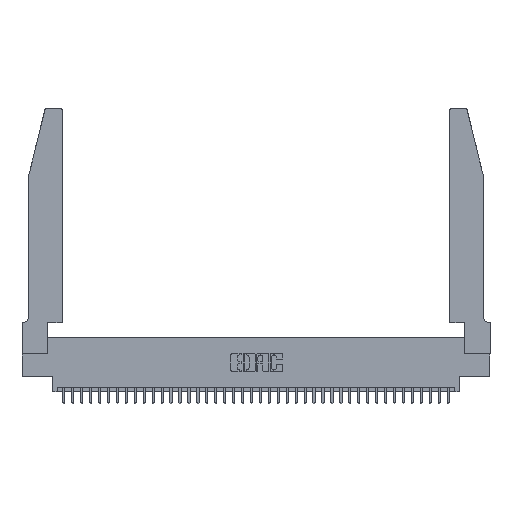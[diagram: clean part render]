
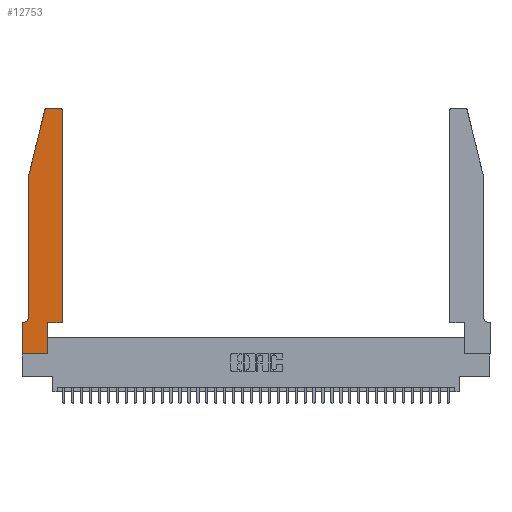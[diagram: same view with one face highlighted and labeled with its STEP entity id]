
A CAD part, top view. The second image highlights one B-rep face of the part: STEP entity #12753.
In plain terms, the highlighted planar face has unit normal (0, 0, 1).
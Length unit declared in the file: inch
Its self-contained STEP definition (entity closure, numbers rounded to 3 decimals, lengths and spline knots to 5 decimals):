
#182 = VECTOR ( 'NONE', #33319, 39.37008 ) ;
#279 = EDGE_CURVE ( 'NONE', #15512, #21603, #10615, .T. ) ;
#410 = DIRECTION ( 'NONE',  ( 1., 0., 0. ) ) ;
#689 = DIRECTION ( 'NONE',  ( 0., 0., 1. ) ) ;
#1297 = EDGE_CURVE ( 'NONE', #25329, #8774, #26705, .T. ) ;
#1304 = CARTESIAN_POINT ( 'NONE',  ( 0.0755, 2., 0.37 ) ) ;
#1874 = EDGE_CURVE ( 'NONE', #21657, #29614, #26146, .T. ) ;
#3122 = ORIENTED_EDGE ( 'NONE', *, *, #33252, .T. ) ;
#4706 = DIRECTION ( 'NONE',  ( 1., 0., 0. ) ) ;
#5196 = EDGE_LOOP ( 'NONE', ( #27425, #20992, #29736, #27773, #10238, #21027, #29947, #9993, #3122, #22848, #13541, #28700 ) ) ;
#5356 = DIRECTION ( 'NONE',  ( 1., 0., 0. ) ) ;
#5960 = AXIS2_PLACEMENT_3D ( 'NONE', #9141, #24368, #410 ) ;
#5963 = CARTESIAN_POINT ( 'NONE',  ( 0.0755, 0.35, 0.37 ) ) ;
#6253 = DIRECTION ( 'NONE',  ( 1., 0., 0. ) ) ;
#6362 = PLANE ( 'NONE',  #5960 ) ;
#7194 = CARTESIAN_POINT ( 'NONE',  ( 0.0755, 2., 0.37 ) ) ;
#7942 = VECTOR ( 'NONE', #10028, 39.37008 ) ;
#8774 = VERTEX_POINT ( 'NONE', #23199 ) ;
#9093 = CARTESIAN_POINT ( 'NONE',  ( 0., 0., 0.37 ) ) ;
#9141 = CARTESIAN_POINT ( 'NONE',  ( 0., 0.35, 0.37 ) ) ;
#9427 = CARTESIAN_POINT ( 'NONE',  ( 0.0755, 2., 0.37 ) ) ;
#9993 = ORIENTED_EDGE ( 'NONE', *, *, #1297, .T. ) ;
#10028 = DIRECTION ( 'NONE',  ( 0., 1., 0. ) ) ;
#10153 = CARTESIAN_POINT ( 'NONE',  ( 0.0755, 0.42, 0.37 ) ) ;
#10203 = AXIS2_PLACEMENT_3D ( 'NONE', #34656, #17429, #23490 ) ;
#10238 = ORIENTED_EDGE ( 'NONE', *, *, #11694, .T. ) ;
#10490 = VERTEX_POINT ( 'NONE', #22959 ) ;
#10532 = CARTESIAN_POINT ( 'NONE',  ( 0.2605, 2.75, 0.37 ) ) ;
#10615 = LINE ( 'NONE', #5963, #16751 ) ;
#11694 = EDGE_CURVE ( 'NONE', #26914, #15512, #14439, .T. ) ;
#11916 = DIRECTION ( 'NONE',  ( -1., 0., 0. ) ) ;
#12753 = ADVANCED_FACE ( 'NONE', ( #20498 ), #6362, .T. ) ;
#13520 = CARTESIAN_POINT ( 'NONE',  ( 0.0055, 0.35, 0.37 ) ) ;
#13541 = ORIENTED_EDGE ( 'NONE', *, *, #35552, .T. ) ;
#14439 = CIRCLE ( 'NONE', #10203, 0.07 ) ;
#15064 = DIRECTION ( 'NONE',  ( 1., 0., 0. ) ) ;
#15512 = VERTEX_POINT ( 'NONE', #13520 ) ;
#15790 = CARTESIAN_POINT ( 'NONE',  ( 0., 0., 0.37 ) ) ;
#15930 = VECTOR ( 'NONE', #25744, 39.37008 ) ;
#16115 = CARTESIAN_POINT ( 'NONE',  ( 0.4505, 0.35, 0.37 ) ) ;
#16228 = LINE ( 'NONE', #9427, #182 ) ;
#16472 = LINE ( 'NONE', #15790, #30693 ) ;
#16525 = VERTEX_POINT ( 'NONE', #7194 ) ;
#16751 = VECTOR ( 'NONE', #11916, 39.37008 ) ;
#16918 = LINE ( 'NONE', #10532, #15930 ) ;
#17429 = DIRECTION ( 'NONE',  ( 0., 0., -1. ) ) ;
#19168 = LINE ( 'NONE', #34633, #34395 ) ;
#20344 = EDGE_CURVE ( 'NONE', #37781, #25888, #33863, .T. ) ;
#20498 = FACE_OUTER_BOUND ( 'NONE', #5196, .T. ) ;
#20985 = VECTOR ( 'NONE', #5356, 39.37008 ) ;
#20992 = ORIENTED_EDGE ( 'NONE', *, *, #20344, .T. ) ;
#21027 = ORIENTED_EDGE ( 'NONE', *, *, #279, .T. ) ;
#21181 = LINE ( 'NONE', #28347, #7942 ) ;
#21559 = CARTESIAN_POINT ( 'NONE',  ( 0.284, 2.72, 0.37 ) ) ;
#21603 = VERTEX_POINT ( 'NONE', #30652 ) ;
#21657 = VERTEX_POINT ( 'NONE', #33522 ) ;
#21779 = DIRECTION ( 'NONE',  ( -0.239, -0.971, 0. ) ) ;
#21870 = EDGE_CURVE ( 'NONE', #25888, #16525, #33797, .T. ) ;
#22848 = ORIENTED_EDGE ( 'NONE', *, *, #34962, .T. ) ;
#22959 = CARTESIAN_POINT ( 'NONE',  ( 0.2865, 0.35, 0.37 ) ) ;
#23199 = CARTESIAN_POINT ( 'NONE',  ( 0.2865, 0., 0.37 ) ) ;
#23490 = DIRECTION ( 'NONE',  ( -1., 0., 0. ) ) ;
#23835 = AXIS2_PLACEMENT_3D ( 'NONE', #21559, #689, #6253 ) ;
#24368 = DIRECTION ( 'NONE',  ( 0., 0., 1. ) ) ;
#24633 = EDGE_CURVE ( 'NONE', #21603, #25329, #16472, .T. ) ;
#24757 = VECTOR ( 'NONE', #21779, 39.37008 ) ;
#25329 = VERTEX_POINT ( 'NONE', #9093 ) ;
#25495 = EDGE_CURVE ( 'NONE', #29614, #37781, #16918, .T. ) ;
#25744 = DIRECTION ( 'NONE',  ( -1., 0., 0. ) ) ;
#25848 = VERTEX_POINT ( 'NONE', #39024 ) ;
#25888 = VERTEX_POINT ( 'NONE', #38757 ) ;
#26146 = CIRCLE ( 'NONE', #27770, 0.03 ) ;
#26705 = LINE ( 'NONE', #35459, #20985 ) ;
#26914 = VERTEX_POINT ( 'NONE', #10153 ) ;
#27361 = CARTESIAN_POINT ( 'NONE',  ( 0.4205, 2.72, 0.37 ) ) ;
#27425 = ORIENTED_EDGE ( 'NONE', *, *, #25495, .T. ) ;
#27483 = DIRECTION ( 'NONE',  ( 0., -1., 0. ) ) ;
#27684 = VECTOR ( 'NONE', #31091, 39.37008 ) ;
#27770 = AXIS2_PLACEMENT_3D ( 'NONE', #27361, #33202, #15064 ) ;
#27773 = ORIENTED_EDGE ( 'NONE', *, *, #32510, .T. ) ;
#28347 = CARTESIAN_POINT ( 'NONE',  ( 0.2865, 0.35, 0.37 ) ) ;
#28700 = ORIENTED_EDGE ( 'NONE', *, *, #1874, .T. ) ;
#29614 = VERTEX_POINT ( 'NONE', #37023 ) ;
#29736 = ORIENTED_EDGE ( 'NONE', *, *, #21870, .T. ) ;
#29947 = ORIENTED_EDGE ( 'NONE', *, *, #24633, .T. ) ;
#30652 = CARTESIAN_POINT ( 'NONE',  ( 0., 0.35, 0.37 ) ) ;
#30693 = VECTOR ( 'NONE', #27483, 39.37008 ) ;
#31091 = DIRECTION ( 'NONE',  ( 0., 1., 0. ) ) ;
#32315 = CARTESIAN_POINT ( 'NONE',  ( 0.284, 2.75, 0.37 ) ) ;
#32510 = EDGE_CURVE ( 'NONE', #16525, #26914, #16228, .T. ) ;
#33202 = DIRECTION ( 'NONE',  ( 0., 0., 1. ) ) ;
#33252 = EDGE_CURVE ( 'NONE', #8774, #10490, #21181, .T. ) ;
#33319 = DIRECTION ( 'NONE',  ( 0., -1., 0. ) ) ;
#33420 = LINE ( 'NONE', #16115, #27684 ) ;
#33522 = CARTESIAN_POINT ( 'NONE',  ( 0.4505, 2.72, 0.37 ) ) ;
#33797 = LINE ( 'NONE', #1304, #24757 ) ;
#33863 = CIRCLE ( 'NONE', #23835, 0.03 ) ;
#34395 = VECTOR ( 'NONE', #4706, 39.37008 ) ;
#34633 = CARTESIAN_POINT ( 'NONE',  ( 0.4505, 0.35, 0.37 ) ) ;
#34656 = CARTESIAN_POINT ( 'NONE',  ( 0.0055, 0.42, 0.37 ) ) ;
#34962 = EDGE_CURVE ( 'NONE', #10490, #25848, #19168, .T. ) ;
#35459 = CARTESIAN_POINT ( 'NONE',  ( 0., 0., 0.37 ) ) ;
#35552 = EDGE_CURVE ( 'NONE', #25848, #21657, #33420, .T. ) ;
#37023 = CARTESIAN_POINT ( 'NONE',  ( 0.4205, 2.75, 0.37 ) ) ;
#37781 = VERTEX_POINT ( 'NONE', #32315 ) ;
#38757 = CARTESIAN_POINT ( 'NONE',  ( 0.25487, 2.72718, 0.37 ) ) ;
#39024 = CARTESIAN_POINT ( 'NONE',  ( 0.4505, 0.35, 0.37 ) ) ;
